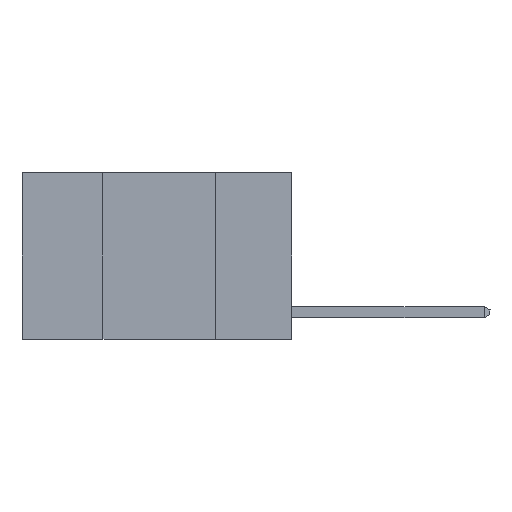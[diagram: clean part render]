
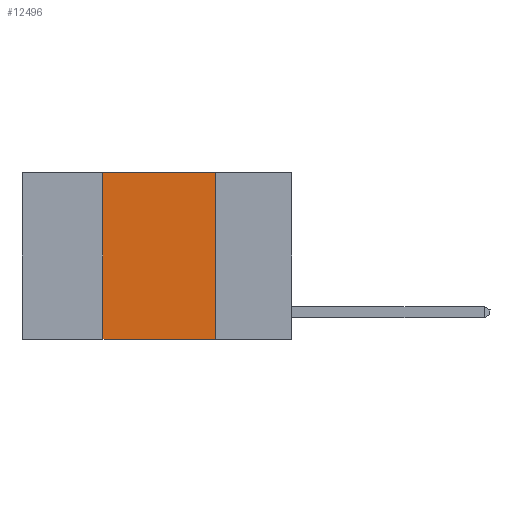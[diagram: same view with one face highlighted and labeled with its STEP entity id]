
A CAD part, left-side view. The second image highlights one B-rep face of the part: STEP entity #12496.
In plain terms, the highlighted planar face has unit normal (-1, 0, 0).
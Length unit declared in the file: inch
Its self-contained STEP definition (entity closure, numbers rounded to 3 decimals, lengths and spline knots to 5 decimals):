
#659 = VERTEX_POINT ( 'NONE', #7022 ) ;
#1414 = VERTEX_POINT ( 'NONE', #10560 ) ;
#1653 = LINE ( 'NONE', #2451, #11522 ) ;
#2451 = CARTESIAN_POINT ( 'NONE',  ( 0., 0.17, 0. ) ) ;
#2993 = ORIENTED_EDGE ( 'NONE', *, *, #10164, .F. ) ;
#3305 = ORIENTED_EDGE ( 'NONE', *, *, #4797, .F. ) ;
#3700 = VERTEX_POINT ( 'NONE', #3761 ) ;
#3761 = CARTESIAN_POINT ( 'NONE',  ( 0., 0.17, -0.37 ) ) ;
#4039 = DIRECTION ( 'NONE',  ( 0., -1., 0. ) ) ;
#4797 = EDGE_CURVE ( 'NONE', #1414, #659, #6828, .T. ) ;
#5321 = LINE ( 'NONE', #6663, #10219 ) ;
#5396 = CARTESIAN_POINT ( 'NONE',  ( 0., 0.17, 0. ) ) ;
#5636 = CARTESIAN_POINT ( 'NONE',  ( 0., 0.6, 0. ) ) ;
#5686 = ORIENTED_EDGE ( 'NONE', *, *, #12711, .F. ) ;
#5984 = ORIENTED_EDGE ( 'NONE', *, *, #8734, .T. ) ;
#6311 = FACE_OUTER_BOUND ( 'NONE', #8098, .T. ) ;
#6606 = DIRECTION ( 'NONE',  ( 0., 0., -1. ) ) ;
#6663 = CARTESIAN_POINT ( 'NONE',  ( 0., 0.6, -0.37 ) ) ;
#6828 = LINE ( 'NONE', #11720, #9091 ) ;
#6909 = DIRECTION ( 'NONE',  ( 0., 0., 1. ) ) ;
#7022 = CARTESIAN_POINT ( 'NONE',  ( 0., 0.42, 0. ) ) ;
#7711 = VERTEX_POINT ( 'NONE', #5396 ) ;
#7994 = CARTESIAN_POINT ( 'NONE',  ( 0., 0.6, 0. ) ) ;
#8074 = AXIS2_PLACEMENT_3D ( 'NONE', #5636, #12396, #6606 ) ;
#8098 = EDGE_LOOP ( 'NONE', ( #2993, #5686, #3305, #5984 ) ) ;
#8734 = EDGE_CURVE ( 'NONE', #1414, #3700, #5321, .T. ) ;
#9047 = VECTOR ( 'NONE', #4039, 39.37008 ) ;
#9091 = VECTOR ( 'NONE', #6909, 39.37008 ) ;
#10164 = EDGE_CURVE ( 'NONE', #7711, #3700, #1653, .T. ) ;
#10219 = VECTOR ( 'NONE', #12441, 39.37008 ) ;
#10364 = DIRECTION ( 'NONE',  ( 0., 0., -1. ) ) ;
#10560 = CARTESIAN_POINT ( 'NONE',  ( 0., 0.42, -0.37 ) ) ;
#11439 = PLANE ( 'NONE',  #8074 ) ;
#11522 = VECTOR ( 'NONE', #10364, 39.37008 ) ;
#11611 = LINE ( 'NONE', #7994, #9047 ) ;
#11720 = CARTESIAN_POINT ( 'NONE',  ( 0., 0.42, 0. ) ) ;
#12396 = DIRECTION ( 'NONE',  ( 1., 0., 0. ) ) ;
#12441 = DIRECTION ( 'NONE',  ( 0., -1., 0. ) ) ;
#12496 = ADVANCED_FACE ( 'NONE', ( #6311 ), #11439, .F. ) ;
#12711 = EDGE_CURVE ( 'NONE', #659, #7711, #11611, .T. ) ;
